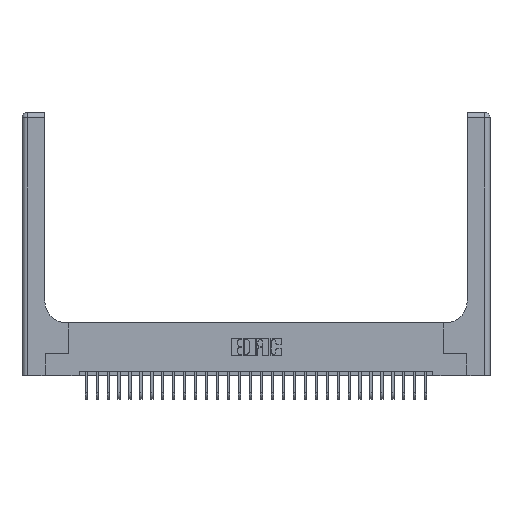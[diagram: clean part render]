
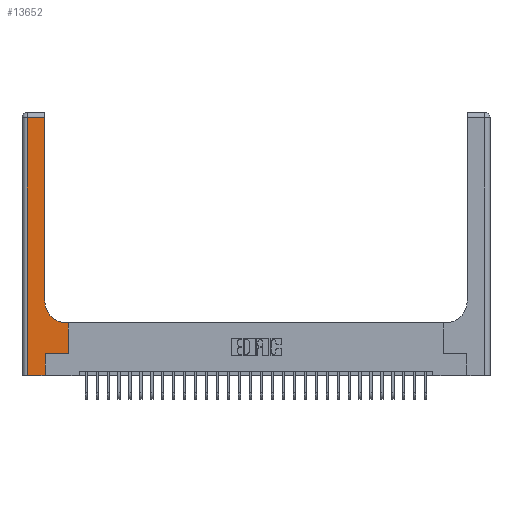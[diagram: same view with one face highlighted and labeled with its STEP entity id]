
A CAD part, top view. The second image highlights one B-rep face of the part: STEP entity #13652.
In plain terms, the highlighted planar face has unit normal (0, 0, 1).
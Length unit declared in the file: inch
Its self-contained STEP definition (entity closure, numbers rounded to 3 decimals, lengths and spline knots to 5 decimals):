
#127 = EDGE_CURVE ( 'NONE', #6526, #13673, #14067, .T. ) ;
#460 = DIRECTION ( 'NONE',  ( -1., 0., 0. ) ) ;
#505 = VERTEX_POINT ( 'NONE', #24091 ) ;
#1797 = CARTESIAN_POINT ( 'NONE',  ( 0.06, 2.94, 0.37 ) ) ;
#2319 = VERTEX_POINT ( 'NONE', #7989 ) ;
#2344 = VERTEX_POINT ( 'NONE', #18141 ) ;
#2497 = CARTESIAN_POINT ( 'NONE',  ( 0.26, 0.6, 0.37 ) ) ;
#3498 = EDGE_CURVE ( 'NONE', #20307, #24383, #12599, .T. ) ;
#3546 = CARTESIAN_POINT ( 'NONE',  ( 0.528, 0.25, 0.37 ) ) ;
#3656 = CARTESIAN_POINT ( 'NONE',  ( 0.26, 3., 0.37 ) ) ;
#4411 = DIRECTION ( 'NONE',  ( 0., 0., -1. ) ) ;
#4730 = CARTESIAN_POINT ( 'NONE',  ( 0.265, 0.25, 0.37 ) ) ;
#4946 = ORIENTED_EDGE ( 'NONE', *, *, #13471, .T. ) ;
#5695 = ORIENTED_EDGE ( 'NONE', *, *, #3498, .T. ) ;
#6261 = CARTESIAN_POINT ( 'NONE',  ( 0., 2.94, 0.37 ) ) ;
#6298 = VECTOR ( 'NONE', #21079, 39.37008 ) ;
#6526 = VERTEX_POINT ( 'NONE', #15866 ) ;
#6823 = EDGE_CURVE ( 'NONE', #13673, #505, #12427, .T. ) ;
#6999 = CARTESIAN_POINT ( 'NONE',  ( 0.265, 0., 0.37 ) ) ;
#7612 = FACE_OUTER_BOUND ( 'NONE', #17198, .T. ) ;
#7687 = ORIENTED_EDGE ( 'NONE', *, *, #13714, .T. ) ;
#7989 = CARTESIAN_POINT ( 'NONE',  ( 0.06, 0., 0.37 ) ) ;
#8397 = VERTEX_POINT ( 'NONE', #19651 ) ;
#8405 = LINE ( 'NONE', #3546, #12581 ) ;
#9970 = CARTESIAN_POINT ( 'NONE',  ( 0.06, 3., 0.37 ) ) ;
#10857 = CARTESIAN_POINT ( 'NONE',  ( 0., 3., 0.37 ) ) ;
#11513 = LINE ( 'NONE', #3656, #16876 ) ;
#11826 = LINE ( 'NONE', #4730, #6298 ) ;
#12427 = CIRCLE ( 'NONE', #20572, 0.25 ) ;
#12581 = VECTOR ( 'NONE', #23970, 39.37008 ) ;
#12599 = LINE ( 'NONE', #6261, #18587 ) ;
#12906 = DIRECTION ( 'NONE',  ( 0., 0., -1. ) ) ;
#13141 = ORIENTED_EDGE ( 'NONE', *, *, #21482, .T. ) ;
#13471 = EDGE_CURVE ( 'NONE', #505, #20307, #11513, .T. ) ;
#13652 = ADVANCED_FACE ( 'NONE', ( #7612 ), #22911, .F. ) ;
#13673 = VERTEX_POINT ( 'NONE', #23006 ) ;
#13714 = EDGE_CURVE ( 'NONE', #8397, #15105, #11826, .T. ) ;
#13737 = VECTOR ( 'NONE', #14777, 39.37008 ) ;
#13783 = ORIENTED_EDGE ( 'NONE', *, *, #22488, .T. ) ;
#14067 = LINE ( 'NONE', #2497, #24754 ) ;
#14475 = CARTESIAN_POINT ( 'NONE',  ( 0.26, 2.94, 0.37 ) ) ;
#14777 = DIRECTION ( 'NONE',  ( 1., 0., 0. ) ) ;
#14873 = EDGE_CURVE ( 'NONE', #2344, #8397, #20883, .T. ) ;
#15105 = VERTEX_POINT ( 'NONE', #15949 ) ;
#15531 = VECTOR ( 'NONE', #19286, 39.37008 ) ;
#15866 = CARTESIAN_POINT ( 'NONE',  ( 0.528, 0.6, 0.37 ) ) ;
#15949 = CARTESIAN_POINT ( 'NONE',  ( 0.528, 0.25, 0.37 ) ) ;
#15995 = DIRECTION ( 'NONE',  ( 0., 1., 0. ) ) ;
#16740 = CARTESIAN_POINT ( 'NONE',  ( 0.51, 0.85, 0.37 ) ) ;
#16800 = AXIS2_PLACEMENT_3D ( 'NONE', #10857, #12906, #460 ) ;
#16820 = CARTESIAN_POINT ( 'NONE',  ( 0., 0., 0.37 ) ) ;
#16876 = VECTOR ( 'NONE', #15995, 39.37008 ) ;
#16911 = DIRECTION ( 'NONE',  ( -1., 0., 0. ) ) ;
#17198 = EDGE_LOOP ( 'NONE', ( #4946, #5695, #23192, #13141, #19756, #7687, #13783, #18358, #18328 ) ) ;
#18141 = CARTESIAN_POINT ( 'NONE',  ( 0.265, 0., 0.37 ) ) ;
#18328 = ORIENTED_EDGE ( 'NONE', *, *, #6823, .T. ) ;
#18358 = ORIENTED_EDGE ( 'NONE', *, *, #127, .T. ) ;
#18587 = VECTOR ( 'NONE', #20513, 39.37008 ) ;
#18748 = DIRECTION ( 'NONE',  ( 1., 0., 0. ) ) ;
#19286 = DIRECTION ( 'NONE',  ( 0., 1., 0. ) ) ;
#19450 = VECTOR ( 'NONE', #24046, 39.37008 ) ;
#19651 = CARTESIAN_POINT ( 'NONE',  ( 0.265, 0.25, 0.37 ) ) ;
#19756 = ORIENTED_EDGE ( 'NONE', *, *, #14873, .T. ) ;
#20307 = VERTEX_POINT ( 'NONE', #14475 ) ;
#20513 = DIRECTION ( 'NONE',  ( -1., 0., 0. ) ) ;
#20572 = AXIS2_PLACEMENT_3D ( 'NONE', #16740, #4411, #18748 ) ;
#20883 = LINE ( 'NONE', #6999, #15531 ) ;
#21079 = DIRECTION ( 'NONE',  ( 1., 0., 0. ) ) ;
#21482 = EDGE_CURVE ( 'NONE', #2319, #2344, #24424, .T. ) ;
#22488 = EDGE_CURVE ( 'NONE', #15105, #6526, #8405, .T. ) ;
#22911 = PLANE ( 'NONE',  #16800 ) ;
#23006 = CARTESIAN_POINT ( 'NONE',  ( 0.51, 0.6, 0.37 ) ) ;
#23192 = ORIENTED_EDGE ( 'NONE', *, *, #24298, .T. ) ;
#23970 = DIRECTION ( 'NONE',  ( 0., 1., 0. ) ) ;
#24046 = DIRECTION ( 'NONE',  ( 0., -1., 0. ) ) ;
#24091 = CARTESIAN_POINT ( 'NONE',  ( 0.26, 0.85, 0.37 ) ) ;
#24168 = LINE ( 'NONE', #9970, #19450 ) ;
#24298 = EDGE_CURVE ( 'NONE', #24383, #2319, #24168, .T. ) ;
#24383 = VERTEX_POINT ( 'NONE', #1797 ) ;
#24424 = LINE ( 'NONE', #16820, #13737 ) ;
#24754 = VECTOR ( 'NONE', #16911, 39.37008 ) ;
